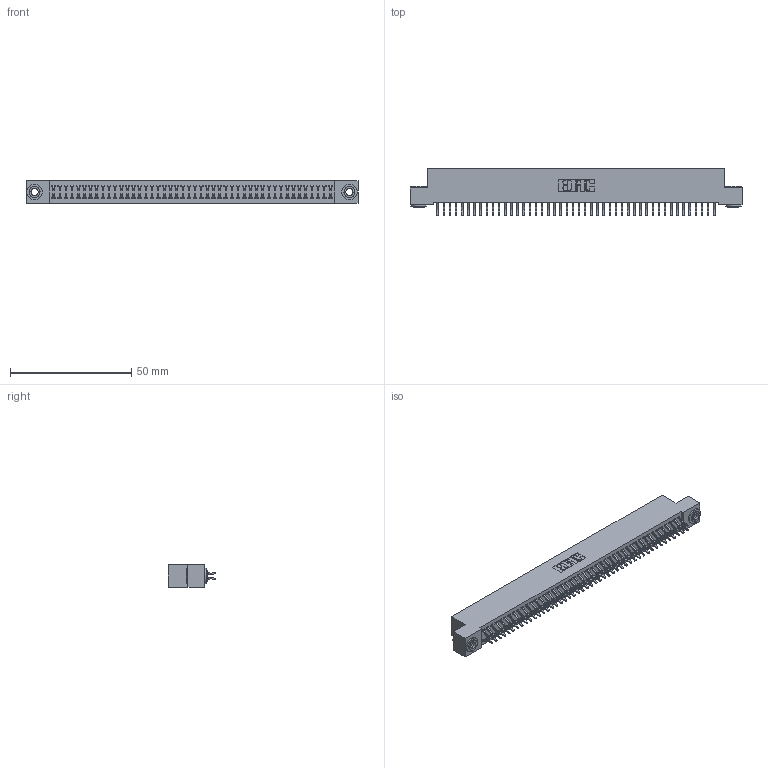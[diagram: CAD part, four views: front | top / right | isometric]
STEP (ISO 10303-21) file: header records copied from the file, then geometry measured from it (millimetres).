
FILE_DESCRIPTION (( 'STEP AP203' ), '1' );
FILE_NAME ('342-092-556-203.STEP', '2019-10-04T15:02:11', ( '' ), ( '' ), 'SwSTEP 2.0', 'SolidWorks 2016', '' );
FILE_SCHEMA (( 'CONFIG_CONTROL_DESIGN' ));
Length unit declared in the file: inch
Products named in the file (4): 345-292-001_556 Tail; 342-250-002_345-250-002-102; 342-092-556-203; 342 Part_.156 TH
Assembly tree (95 placements, depth 2):
  342-092-556-203
    342 Part_.156 TH
    345-292-001_556 Tail  x92
    342-250-002_345-250-002-102  x2
Bounding box: 137.16 x 19.58 x 9.4 mm (x, y, z)
Volume: 12363.2 mm3; surface area: 20347.6 mm2
Topology: 95 solids, 95 shells, 5484 faces, 16291 edges, 10734 vertices
Faces by surface type: plane 3756, cylinder 1720, cone 8
Entity records: 29814 total; most frequent: CARTESIAN_POINT 4925, ORIENTED_EDGE 4842, DIRECTION 4223, EDGE_CURVE 2421, VECTOR 2261, LINE 2261, VERTEX_POINT 1610, AXIS2_PLACEMENT_3D 981
